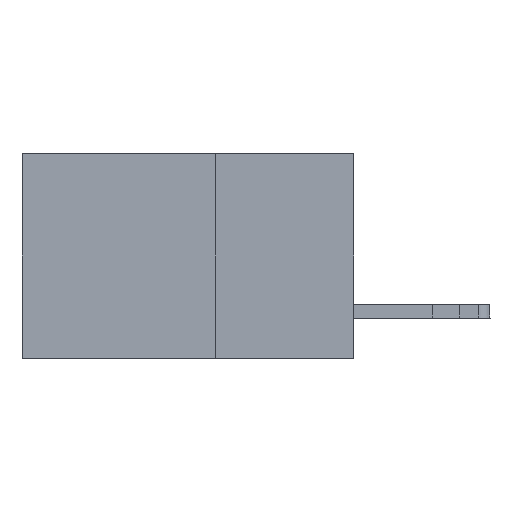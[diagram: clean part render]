
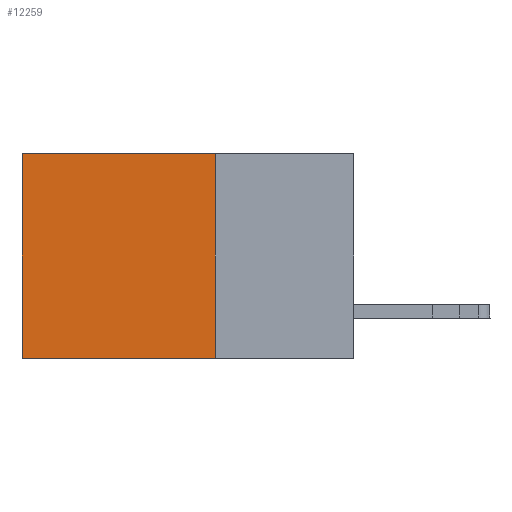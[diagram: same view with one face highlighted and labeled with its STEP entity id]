
A CAD part, left-side view. The second image highlights one B-rep face of the part: STEP entity #12259.
In plain terms, the highlighted planar face has unit normal (-1, 0, 0).
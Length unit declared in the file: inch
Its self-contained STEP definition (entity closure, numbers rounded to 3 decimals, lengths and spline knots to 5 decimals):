
#1313 = LINE ( 'NONE', #22080, #2231 ) ;
#1943 = EDGE_LOOP ( 'NONE', ( #5752, #24926, #28692, #26584 ) ) ;
#2231 = VECTOR ( 'NONE', #3969, 39.37008 ) ;
#3371 = AXIS2_PLACEMENT_3D ( 'NONE', #24726, #27704, #9642 ) ;
#3547 = VERTEX_POINT ( 'NONE', #21621 ) ;
#3570 = PLANE ( 'NONE',  #3371 ) ;
#3703 = VERTEX_POINT ( 'NONE', #10222 ) ;
#3969 = DIRECTION ( 'NONE',  ( 0., 0., -1. ) ) ;
#4750 = EDGE_CURVE ( 'NONE', #32279, #3703, #20191, .T. ) ;
#5752 = ORIENTED_EDGE ( 'NONE', *, *, #31051, .T. ) ;
#7073 = CARTESIAN_POINT ( 'NONE',  ( 0.2875, 0.25, -0.37 ) ) ;
#7636 = VECTOR ( 'NONE', #27578, 39.37008 ) ;
#8567 = LINE ( 'NONE', #15647, #7636 ) ;
#9642 = DIRECTION ( 'NONE',  ( 0., 0., -1. ) ) ;
#9783 = CARTESIAN_POINT ( 'NONE',  ( 0.2875, 0.25, 0. ) ) ;
#10222 = CARTESIAN_POINT ( 'NONE',  ( 0.2875, 0.25, -0.37 ) ) ;
#11673 = EDGE_CURVE ( 'NONE', #3703, #36353, #28915, .T. ) ;
#12259 = ADVANCED_FACE ( 'NONE', ( #24199 ), #3570, .F. ) ;
#15647 = CARTESIAN_POINT ( 'NONE',  ( 0.2875, 0.25, 0. ) ) ;
#15847 = DIRECTION ( 'NONE',  ( 0., 0., -1. ) ) ;
#15964 = VECTOR ( 'NONE', #15847, 39.37008 ) ;
#20191 = LINE ( 'NONE', #33841, #15964 ) ;
#21621 = CARTESIAN_POINT ( 'NONE',  ( 0.2875, 0.6, 0. ) ) ;
#22080 = CARTESIAN_POINT ( 'NONE',  ( 0.2875, 0.6, 0. ) ) ;
#24199 = FACE_OUTER_BOUND ( 'NONE', #1943, .T. ) ;
#24726 = CARTESIAN_POINT ( 'NONE',  ( 0.2875, 0.25, 0. ) ) ;
#24926 = ORIENTED_EDGE ( 'NONE', *, *, #11673, .F. ) ;
#26584 = ORIENTED_EDGE ( 'NONE', *, *, #34174, .T. ) ;
#27578 = DIRECTION ( 'NONE',  ( 0., 1., 0. ) ) ;
#27704 = DIRECTION ( 'NONE',  ( 1., 0., 0. ) ) ;
#28144 = DIRECTION ( 'NONE',  ( 0., 1., 0. ) ) ;
#28692 = ORIENTED_EDGE ( 'NONE', *, *, #4750, .F. ) ;
#28915 = LINE ( 'NONE', #7073, #36846 ) ;
#28996 = CARTESIAN_POINT ( 'NONE',  ( 0.2875, 0.6, -0.37 ) ) ;
#31051 = EDGE_CURVE ( 'NONE', #3547, #36353, #1313, .T. ) ;
#32279 = VERTEX_POINT ( 'NONE', #9783 ) ;
#33841 = CARTESIAN_POINT ( 'NONE',  ( 0.2875, 0.25, 0. ) ) ;
#34174 = EDGE_CURVE ( 'NONE', #32279, #3547, #8567, .T. ) ;
#36353 = VERTEX_POINT ( 'NONE', #28996 ) ;
#36846 = VECTOR ( 'NONE', #28144, 39.37008 ) ;
